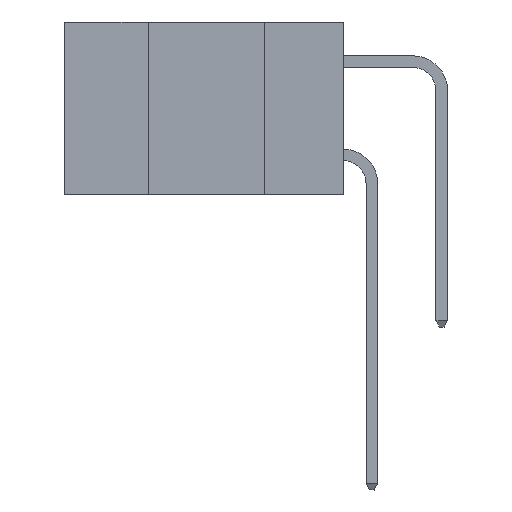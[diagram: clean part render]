
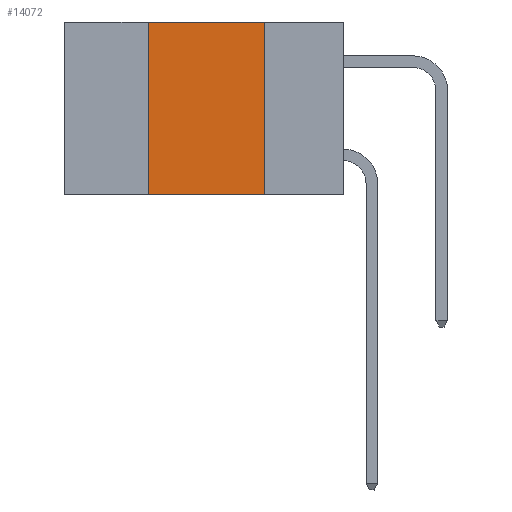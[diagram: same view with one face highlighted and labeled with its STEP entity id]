
A CAD part, left-side view. The second image highlights one B-rep face of the part: STEP entity #14072.
In plain terms, the highlighted planar face has unit normal (-1, 0, 0).
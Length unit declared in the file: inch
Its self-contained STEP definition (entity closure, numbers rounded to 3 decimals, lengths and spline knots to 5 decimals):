
#131 = DIRECTION ( 'NONE',  ( 0., -1., 0. ) ) ;
#1233 = CARTESIAN_POINT ( 'NONE',  ( 0., 0.6, 0. ) ) ;
#1494 = VERTEX_POINT ( 'NONE', #7503 ) ;
#2906 = ORIENTED_EDGE ( 'NONE', *, *, #3996, .F. ) ;
#3688 = EDGE_CURVE ( 'NONE', #1494, #11607, #8779, .T. ) ;
#3996 = EDGE_CURVE ( 'NONE', #11607, #12922, #9367, .T. ) ;
#4098 = CARTESIAN_POINT ( 'NONE',  ( 0., 0.17, 0. ) ) ;
#4105 = FACE_OUTER_BOUND ( 'NONE', #8783, .T. ) ;
#4255 = ORIENTED_EDGE ( 'NONE', *, *, #3688, .F. ) ;
#4488 = CARTESIAN_POINT ( 'NONE',  ( 0., 0.17, -0.37 ) ) ;
#6632 = PLANE ( 'NONE',  #13678 ) ;
#7500 = VECTOR ( 'NONE', #9403, 39.37008 ) ;
#7503 = CARTESIAN_POINT ( 'NONE',  ( 0., 0.42, -0.37 ) ) ;
#7905 = DIRECTION ( 'NONE',  ( 0., 0., -1. ) ) ;
#8256 = CARTESIAN_POINT ( 'NONE',  ( 0., 0.6, 0. ) ) ;
#8507 = ORIENTED_EDGE ( 'NONE', *, *, #8888, .T. ) ;
#8779 = LINE ( 'NONE', #12047, #17504 ) ;
#8783 = EDGE_LOOP ( 'NONE', ( #10440, #2906, #4255, #8507 ) ) ;
#8848 = EDGE_CURVE ( 'NONE', #12922, #11015, #16209, .T. ) ;
#8888 = EDGE_CURVE ( 'NONE', #1494, #11015, #12149, .T. ) ;
#9367 = LINE ( 'NONE', #8256, #9560 ) ;
#9403 = DIRECTION ( 'NONE',  ( 0., -1., 0. ) ) ;
#9560 = VECTOR ( 'NONE', #131, 39.37008 ) ;
#9806 = CARTESIAN_POINT ( 'NONE',  ( 0., 0.42, 0. ) ) ;
#10255 = VECTOR ( 'NONE', #7905, 39.37008 ) ;
#10440 = ORIENTED_EDGE ( 'NONE', *, *, #8848, .F. ) ;
#10912 = DIRECTION ( 'NONE',  ( 1., 0., 0. ) ) ;
#11015 = VERTEX_POINT ( 'NONE', #4488 ) ;
#11607 = VERTEX_POINT ( 'NONE', #9806 ) ;
#12047 = CARTESIAN_POINT ( 'NONE',  ( 0., 0.42, 0. ) ) ;
#12149 = LINE ( 'NONE', #16176, #7500 ) ;
#12922 = VERTEX_POINT ( 'NONE', #13293 ) ;
#13293 = CARTESIAN_POINT ( 'NONE',  ( 0., 0.17, 0. ) ) ;
#13678 = AXIS2_PLACEMENT_3D ( 'NONE', #1233, #10912, #14730 ) ;
#14072 = ADVANCED_FACE ( 'NONE', ( #4105 ), #6632, .F. ) ;
#14730 = DIRECTION ( 'NONE',  ( 0., 0., -1. ) ) ;
#16163 = DIRECTION ( 'NONE',  ( 0., 0., 1. ) ) ;
#16176 = CARTESIAN_POINT ( 'NONE',  ( 0., 0.6, -0.37 ) ) ;
#16209 = LINE ( 'NONE', #4098, #10255 ) ;
#17504 = VECTOR ( 'NONE', #16163, 39.37008 ) ;
